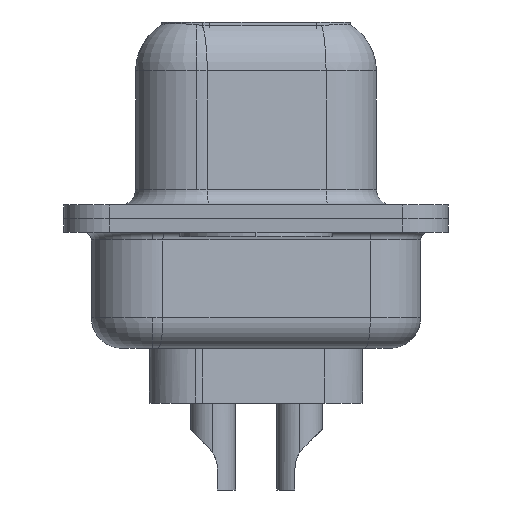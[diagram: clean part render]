
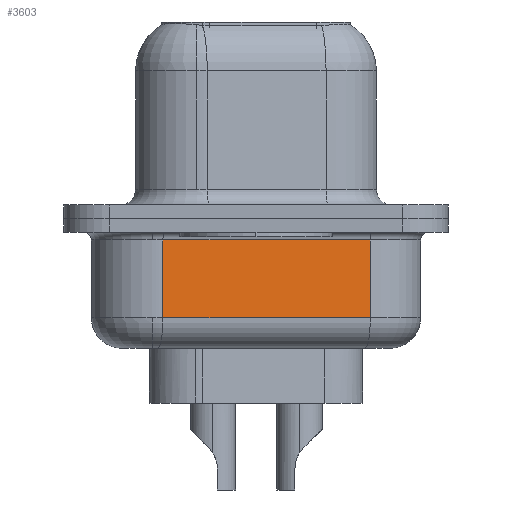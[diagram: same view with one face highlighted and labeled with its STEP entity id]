
A CAD part, left-side view. The second image highlights one B-rep face of the part: STEP entity #3603.
In plain terms, the highlighted planar face has unit normal (-0.985, -0.174, 0).
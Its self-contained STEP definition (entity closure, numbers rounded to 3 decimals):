
#190 = DIRECTION ( 'NONE',  ( -0.174, 0.985, 0. ) ) ;
#197 = LINE ( 'NONE', #9563, #3711 ) ;
#420 = LINE ( 'NONE', #4437, #2353 ) ;
#1220 = ORIENTED_EDGE ( 'NONE', *, *, #11011, .T. ) ;
#1479 = CARTESIAN_POINT ( 'NONE',  ( 2.875, 3.053, -0.7 ) ) ;
#1745 = VECTOR ( 'NONE', #16542, 1000. ) ;
#2092 = CARTESIAN_POINT ( 'NONE',  ( 2.875, 3.053, -0.7 ) ) ;
#2353 = VECTOR ( 'NONE', #9786, 1000. ) ;
#2672 = PLANE ( 'NONE',  #9006 ) ;
#2825 = EDGE_CURVE ( 'NONE', #13437, #11790, #197, .T. ) ;
#3603 = ADVANCED_FACE ( 'NONE', ( #14702 ), #2672, .F. ) ;
#3711 = VECTOR ( 'NONE', #5722, 1000. ) ;
#4437 = CARTESIAN_POINT ( 'NONE',  ( 2.875, 3.053, -3.25 ) ) ;
#4811 = CARTESIAN_POINT ( 'NONE',  ( 4.074, -3.747, -3.25 ) ) ;
#4928 = DIRECTION ( 'NONE',  ( -0.174, 0.985, 0. ) ) ;
#5722 = DIRECTION ( 'NONE',  ( 0., 0., 1. ) ) ;
#6838 = VERTEX_POINT ( 'NONE', #15273 ) ;
#7543 = EDGE_CURVE ( 'NONE', #6838, #7978, #13629, .T. ) ;
#7978 = VERTEX_POINT ( 'NONE', #2092 ) ;
#8545 = CARTESIAN_POINT ( 'NONE',  ( 2.875, 3.053, -4.25 ) ) ;
#9006 = AXIS2_PLACEMENT_3D ( 'NONE', #12743, #16871, #4928 ) ;
#9563 = CARTESIAN_POINT ( 'NONE',  ( 4.074, -3.747, -4.25 ) ) ;
#9786 = DIRECTION ( 'NONE',  ( 0.174, -0.985, 0. ) ) ;
#10865 = LINE ( 'NONE', #1479, #13624 ) ;
#11011 = EDGE_CURVE ( 'NONE', #6838, #13437, #420, .T. ) ;
#11695 = ORIENTED_EDGE ( 'NONE', *, *, #2825, .T. ) ;
#11790 = VERTEX_POINT ( 'NONE', #17195 ) ;
#12743 = CARTESIAN_POINT ( 'NONE',  ( 2.875, 3.053, -4.25 ) ) ;
#13437 = VERTEX_POINT ( 'NONE', #4811 ) ;
#13624 = VECTOR ( 'NONE', #190, 1000. ) ;
#13629 = LINE ( 'NONE', #8545, #1745 ) ;
#14538 = EDGE_CURVE ( 'NONE', #11790, #7978, #10865, .T. ) ;
#14702 = FACE_OUTER_BOUND ( 'NONE', #14730, .T. ) ;
#14730 = EDGE_LOOP ( 'NONE', ( #16034, #1220, #11695, #15779 ) ) ;
#15273 = CARTESIAN_POINT ( 'NONE',  ( 2.875, 3.053, -3.25 ) ) ;
#15779 = ORIENTED_EDGE ( 'NONE', *, *, #14538, .T. ) ;
#16034 = ORIENTED_EDGE ( 'NONE', *, *, #7543, .F. ) ;
#16542 = DIRECTION ( 'NONE',  ( 0., 0., 1. ) ) ;
#16871 = DIRECTION ( 'NONE',  ( 0.985, 0.174, 0. ) ) ;
#17195 = CARTESIAN_POINT ( 'NONE',  ( 4.074, -3.747, -0.7 ) ) ;
